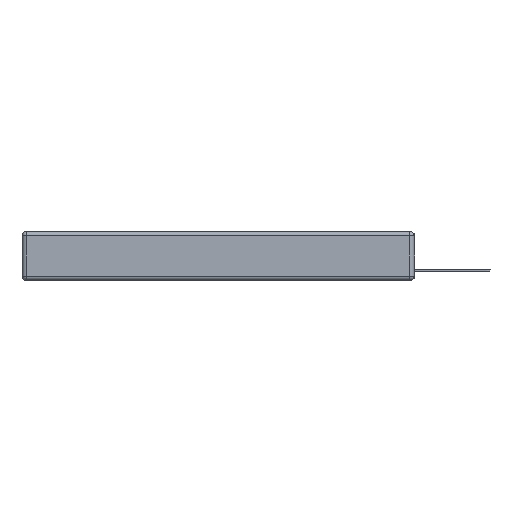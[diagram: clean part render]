
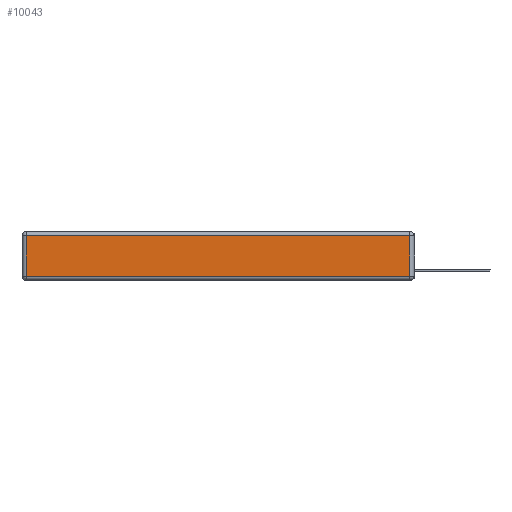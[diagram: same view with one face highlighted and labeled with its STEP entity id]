
A CAD part, left-side view. The second image highlights one B-rep face of the part: STEP entity #10043.
In plain terms, the highlighted planar face has unit normal (-1, 0, 0).
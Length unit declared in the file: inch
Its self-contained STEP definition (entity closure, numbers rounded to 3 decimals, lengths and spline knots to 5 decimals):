
#564 = ORIENTED_EDGE ( 'NONE', *, *, #12032, .T. ) ;
#754 = CARTESIAN_POINT ( 'NONE',  ( 0., 2.72, -0.343 ) ) ;
#1010 = VECTOR ( 'NONE', #8708, 39.37008 ) ;
#1063 = LINE ( 'NONE', #754, #14250 ) ;
#1808 = EDGE_CURVE ( 'NONE', #3859, #11541, #1063, .T. ) ;
#2766 = AXIS2_PLACEMENT_3D ( 'NONE', #15239, #16695, #10927 ) ;
#2976 = VECTOR ( 'NONE', #9919, 39.37008 ) ;
#3482 = ORIENTED_EDGE ( 'NONE', *, *, #10612, .T. ) ;
#3859 = VERTEX_POINT ( 'NONE', #12043 ) ;
#4945 = DIRECTION ( 'NONE',  ( 0., 0., 1. ) ) ;
#5014 = CARTESIAN_POINT ( 'NONE',  ( 0., 0.03, -0.343 ) ) ;
#5741 = CARTESIAN_POINT ( 'NONE',  ( 0., 0.03, -0.03 ) ) ;
#5997 = ORIENTED_EDGE ( 'NONE', *, *, #10639, .T. ) ;
#6220 = VECTOR ( 'NONE', #4945, 39.37008 ) ;
#6509 = FACE_OUTER_BOUND ( 'NONE', #7810, .T. ) ;
#6633 = PLANE ( 'NONE',  #2766 ) ;
#7636 = VERTEX_POINT ( 'NONE', #17521 ) ;
#7754 = LINE ( 'NONE', #5014, #6220 ) ;
#7810 = EDGE_LOOP ( 'NONE', ( #3482, #564, #5997, #12672 ) ) ;
#8708 = DIRECTION ( 'NONE',  ( 0., 1., 0. ) ) ;
#8903 = LINE ( 'NONE', #12739, #2976 ) ;
#9028 = DIRECTION ( 'NONE',  ( 0., 0., -1. ) ) ;
#9559 = LINE ( 'NONE', #15592, #1010 ) ;
#9919 = DIRECTION ( 'NONE',  ( 0., -1., 0. ) ) ;
#10043 = ADVANCED_FACE ( 'NONE', ( #6509 ), #6633, .T. ) ;
#10612 = EDGE_CURVE ( 'NONE', #11541, #7636, #8903, .T. ) ;
#10639 = EDGE_CURVE ( 'NONE', #13311, #3859, #9559, .T. ) ;
#10927 = DIRECTION ( 'NONE',  ( 0., 0., 1. ) ) ;
#11541 = VERTEX_POINT ( 'NONE', #11868 ) ;
#11868 = CARTESIAN_POINT ( 'NONE',  ( 0., 2.72, -0.313 ) ) ;
#12032 = EDGE_CURVE ( 'NONE', #7636, #13311, #7754, .T. ) ;
#12043 = CARTESIAN_POINT ( 'NONE',  ( 0., 2.72, -0.03 ) ) ;
#12672 = ORIENTED_EDGE ( 'NONE', *, *, #1808, .T. ) ;
#12739 = CARTESIAN_POINT ( 'NONE',  ( 0., 0., -0.313 ) ) ;
#13311 = VERTEX_POINT ( 'NONE', #5741 ) ;
#14250 = VECTOR ( 'NONE', #9028, 39.37008 ) ;
#15239 = CARTESIAN_POINT ( 'NONE',  ( 0., 0., -0.343 ) ) ;
#15592 = CARTESIAN_POINT ( 'NONE',  ( 0., 2.75, -0.03 ) ) ;
#16695 = DIRECTION ( 'NONE',  ( -1., 0., 0. ) ) ;
#17521 = CARTESIAN_POINT ( 'NONE',  ( 0., 0.03, -0.313 ) ) ;
